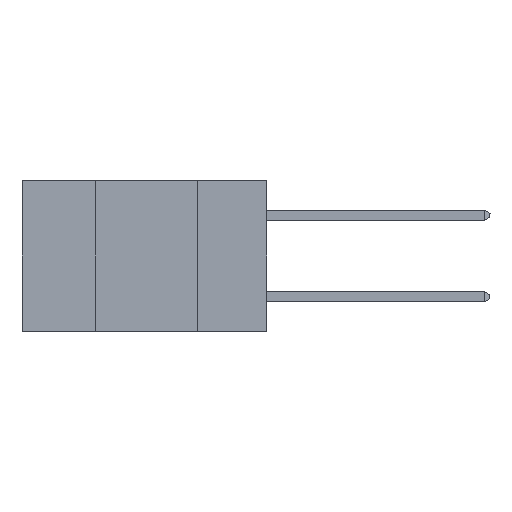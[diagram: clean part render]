
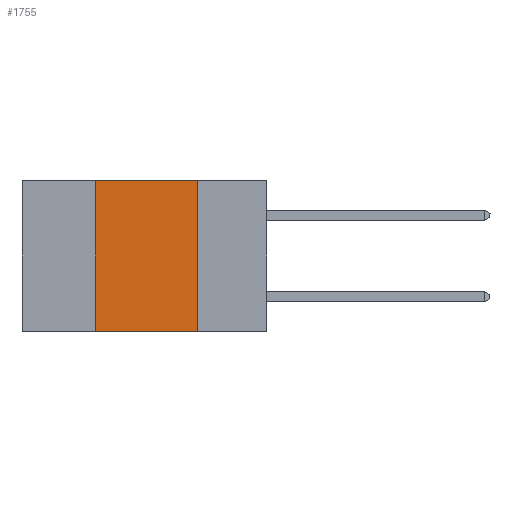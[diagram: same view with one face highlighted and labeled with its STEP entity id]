
A CAD part, left-side view. The second image highlights one B-rep face of the part: STEP entity #1755.
In plain terms, the highlighted planar face has unit normal (-1, 0, 0).
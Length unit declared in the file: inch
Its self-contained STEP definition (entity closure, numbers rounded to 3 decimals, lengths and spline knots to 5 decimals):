
#115 = CARTESIAN_POINT ( 'NONE',  ( 0., 0.42, -0.37 ) ) ;
#597 = ORIENTED_EDGE ( 'NONE', *, *, #10177, .F. ) ;
#810 = ORIENTED_EDGE ( 'NONE', *, *, #12772, .F. ) ;
#1352 = EDGE_LOOP ( 'NONE', ( #597, #810, #12555, #12537 ) ) ;
#1755 = ADVANCED_FACE ( 'NONE', ( #6201 ), #11656, .F. ) ;
#1896 = VECTOR ( 'NONE', #2290, 39.37008 ) ;
#2290 = DIRECTION ( 'NONE',  ( 0., 0., 1. ) ) ;
#2478 = VECTOR ( 'NONE', #5999, 39.37008 ) ;
#3236 = CARTESIAN_POINT ( 'NONE',  ( 0., 0.6, -0.37 ) ) ;
#4176 = LINE ( 'NONE', #7672, #10904 ) ;
#4192 = CARTESIAN_POINT ( 'NONE',  ( 0., 0.17, 0. ) ) ;
#4232 = DIRECTION ( 'NONE',  ( 0., -1., 0. ) ) ;
#4307 = VECTOR ( 'NONE', #4232, 39.37008 ) ;
#4729 = CARTESIAN_POINT ( 'NONE',  ( 0., 0.6, 0. ) ) ;
#4814 = EDGE_CURVE ( 'NONE', #7536, #12081, #7958, .T. ) ;
#5999 = DIRECTION ( 'NONE',  ( 0., 0., -1. ) ) ;
#6201 = FACE_OUTER_BOUND ( 'NONE', #1352, .T. ) ;
#6875 = CARTESIAN_POINT ( 'NONE',  ( 0., 0.42, 0. ) ) ;
#7205 = EDGE_CURVE ( 'NONE', #7536, #7988, #8045, .T. ) ;
#7536 = VERTEX_POINT ( 'NONE', #115 ) ;
#7672 = CARTESIAN_POINT ( 'NONE',  ( 0., 0.6, 0. ) ) ;
#7804 = AXIS2_PLACEMENT_3D ( 'NONE', #4729, #10663, #12583 ) ;
#7878 = CARTESIAN_POINT ( 'NONE',  ( 0., 0.17, -0.37 ) ) ;
#7958 = LINE ( 'NONE', #3236, #4307 ) ;
#7988 = VERTEX_POINT ( 'NONE', #6875 ) ;
#8045 = LINE ( 'NONE', #8310, #1896 ) ;
#8233 = VERTEX_POINT ( 'NONE', #9007 ) ;
#8310 = CARTESIAN_POINT ( 'NONE',  ( 0., 0.42, 0. ) ) ;
#9007 = CARTESIAN_POINT ( 'NONE',  ( 0., 0.17, 0. ) ) ;
#10165 = LINE ( 'NONE', #4192, #2478 ) ;
#10177 = EDGE_CURVE ( 'NONE', #8233, #12081, #10165, .T. ) ;
#10519 = DIRECTION ( 'NONE',  ( 0., -1., 0. ) ) ;
#10663 = DIRECTION ( 'NONE',  ( 1., 0., 0. ) ) ;
#10904 = VECTOR ( 'NONE', #10519, 39.37008 ) ;
#11656 = PLANE ( 'NONE',  #7804 ) ;
#12081 = VERTEX_POINT ( 'NONE', #7878 ) ;
#12537 = ORIENTED_EDGE ( 'NONE', *, *, #4814, .T. ) ;
#12555 = ORIENTED_EDGE ( 'NONE', *, *, #7205, .F. ) ;
#12583 = DIRECTION ( 'NONE',  ( 0., 0., -1. ) ) ;
#12772 = EDGE_CURVE ( 'NONE', #7988, #8233, #4176, .T. ) ;
